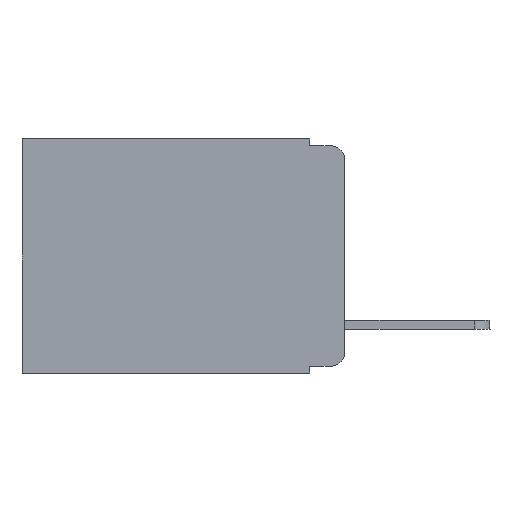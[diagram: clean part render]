
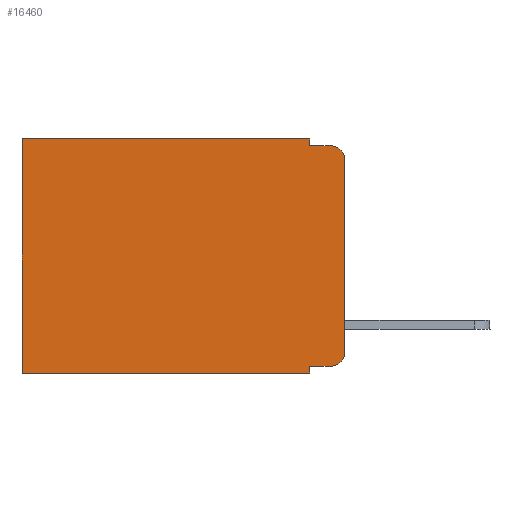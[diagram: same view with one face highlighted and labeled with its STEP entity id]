
A CAD part, left-side view. The second image highlights one B-rep face of the part: STEP entity #16460.
In plain terms, the highlighted planar face has unit normal (-1, 0, 0).
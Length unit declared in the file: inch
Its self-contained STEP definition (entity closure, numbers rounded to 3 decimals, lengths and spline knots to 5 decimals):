
#746 = CIRCLE ( 'NONE', #1974, 0.02 ) ;
#1625 = VERTEX_POINT ( 'NONE', #5108 ) ;
#1913 = CARTESIAN_POINT ( 'NONE',  ( 0.298, 0.02, -0.333 ) ) ;
#1974 = AXIS2_PLACEMENT_3D ( 'NONE', #5790, #13665, #3856 ) ;
#2011 = ORIENTED_EDGE ( 'NONE', *, *, #16342, .T. ) ;
#2152 = CARTESIAN_POINT ( 'NONE',  ( 0.298, 0.051, -0.01 ) ) ;
#2424 = ORIENTED_EDGE ( 'NONE', *, *, #23788, .T. ) ;
#2714 = VERTEX_POINT ( 'NONE', #8242 ) ;
#3777 = VECTOR ( 'NONE', #24983, 39.37008 ) ;
#3856 = DIRECTION ( 'NONE',  ( 0., 0., -1. ) ) ;
#3954 = VECTOR ( 'NONE', #24183, 39.37008 ) ;
#3997 = PLANE ( 'NONE',  #16964 ) ;
#4040 = CARTESIAN_POINT ( 'NONE',  ( 0.298, 0.473, 0. ) ) ;
#4423 = ORIENTED_EDGE ( 'NONE', *, *, #13741, .T. ) ;
#4662 = VECTOR ( 'NONE', #5682, 39.37008 ) ;
#5108 = CARTESIAN_POINT ( 'NONE',  ( 0.298, 0.473, -0.343 ) ) ;
#5442 = VERTEX_POINT ( 'NONE', #7423 ) ;
#5682 = DIRECTION ( 'NONE',  ( 0., -1., 0. ) ) ;
#5790 = CARTESIAN_POINT ( 'NONE',  ( 0.298, 0.02, -0.03 ) ) ;
#6003 = VERTEX_POINT ( 'NONE', #4040 ) ;
#6009 = VECTOR ( 'NONE', #10726, 39.37008 ) ;
#6402 = CIRCLE ( 'NONE', #9710, 0.02 ) ;
#6688 = CARTESIAN_POINT ( 'NONE',  ( 0.298, 0., 0. ) ) ;
#6774 = DIRECTION ( 'NONE',  ( 0., 0., -1. ) ) ;
#7169 = CARTESIAN_POINT ( 'NONE',  ( 0.298, 0., -0.03 ) ) ;
#7273 = VECTOR ( 'NONE', #11265, 39.37008 ) ;
#7423 = CARTESIAN_POINT ( 'NONE',  ( 0.298, 0.051, -0.343 ) ) ;
#7435 = CARTESIAN_POINT ( 'NONE',  ( 0.298, 0., -0.313 ) ) ;
#7509 = DIRECTION ( 'NONE',  ( 0., 0., -1. ) ) ;
#8242 = CARTESIAN_POINT ( 'NONE',  ( 0.298, 0.051, 0. ) ) ;
#8261 = LINE ( 'NONE', #24100, #6009 ) ;
#8814 = EDGE_CURVE ( 'NONE', #17631, #5442, #17061, .T. ) ;
#9164 = VECTOR ( 'NONE', #6774, 39.37008 ) ;
#9539 = FACE_OUTER_BOUND ( 'NONE', #16174, .T. ) ;
#9710 = AXIS2_PLACEMENT_3D ( 'NONE', #15259, #15136, #7509 ) ;
#9766 = CARTESIAN_POINT ( 'NONE',  ( 0.298, 0.02, -0.01 ) ) ;
#9841 = EDGE_CURVE ( 'NONE', #20473, #23531, #746, .T. ) ;
#10006 = LINE ( 'NONE', #14264, #21093 ) ;
#10542 = CARTESIAN_POINT ( 'NONE',  ( 0.298, 0., -0.343 ) ) ;
#10726 = DIRECTION ( 'NONE',  ( 0., 0., -1. ) ) ;
#11265 = DIRECTION ( 'NONE',  ( 0., 0., -1. ) ) ;
#11506 = VERTEX_POINT ( 'NONE', #2152 ) ;
#12406 = ORIENTED_EDGE ( 'NONE', *, *, #17165, .F. ) ;
#12609 = LINE ( 'NONE', #10542, #3954 ) ;
#12883 = LINE ( 'NONE', #6688, #21609 ) ;
#13665 = DIRECTION ( 'NONE',  ( -1., 0., 0. ) ) ;
#13741 = EDGE_CURVE ( 'NONE', #17631, #23526, #23322, .T. ) ;
#14264 = CARTESIAN_POINT ( 'NONE',  ( 0.298, 0.051, -0.01 ) ) ;
#14398 = EDGE_CURVE ( 'NONE', #11506, #23531, #10006, .T. ) ;
#14998 = CARTESIAN_POINT ( 'NONE',  ( 0.298, 0.051, -0.333 ) ) ;
#15136 = DIRECTION ( 'NONE',  ( -1., 0., 0. ) ) ;
#15259 = CARTESIAN_POINT ( 'NONE',  ( 0.298, 0.02, -0.313 ) ) ;
#16174 = EDGE_LOOP ( 'NONE', ( #12406, #21165, #24894, #22397, #22402, #2011, #18410, #25154, #4423, #2424 ) ) ;
#16342 = EDGE_CURVE ( 'NONE', #6003, #1625, #20889, .T. ) ;
#16460 = ADVANCED_FACE ( 'NONE', ( #9539 ), #3997, .F. ) ;
#16953 = LINE ( 'NONE', #22501, #9164 ) ;
#16964 = AXIS2_PLACEMENT_3D ( 'NONE', #19575, #19717, #17522 ) ;
#17061 = LINE ( 'NONE', #18997, #7273 ) ;
#17165 = EDGE_CURVE ( 'NONE', #20473, #21782, #16953, .T. ) ;
#17393 = CARTESIAN_POINT ( 'NONE',  ( 0.298, 0.051, -0.333 ) ) ;
#17522 = DIRECTION ( 'NONE',  ( 0., 0., -1. ) ) ;
#17631 = VERTEX_POINT ( 'NONE', #14998 ) ;
#18410 = ORIENTED_EDGE ( 'NONE', *, *, #20294, .F. ) ;
#18997 = CARTESIAN_POINT ( 'NONE',  ( 0.298, 0.051, 0. ) ) ;
#19575 = CARTESIAN_POINT ( 'NONE',  ( 0.298, 0., 0. ) ) ;
#19696 = EDGE_CURVE ( 'NONE', #2714, #6003, #12883, .T. ) ;
#19717 = DIRECTION ( 'NONE',  ( 1., 0., 0. ) ) ;
#20294 = EDGE_CURVE ( 'NONE', #5442, #1625, #12609, .T. ) ;
#20473 = VERTEX_POINT ( 'NONE', #7169 ) ;
#20889 = LINE ( 'NONE', #21012, #3777 ) ;
#21012 = CARTESIAN_POINT ( 'NONE',  ( 0.298, 0.473, 0. ) ) ;
#21093 = VECTOR ( 'NONE', #22116, 39.37008 ) ;
#21165 = ORIENTED_EDGE ( 'NONE', *, *, #9841, .T. ) ;
#21609 = VECTOR ( 'NONE', #22671, 39.37008 ) ;
#21782 = VERTEX_POINT ( 'NONE', #7435 ) ;
#22116 = DIRECTION ( 'NONE',  ( 0., -1., 0. ) ) ;
#22397 = ORIENTED_EDGE ( 'NONE', *, *, #24111, .F. ) ;
#22402 = ORIENTED_EDGE ( 'NONE', *, *, #19696, .T. ) ;
#22501 = CARTESIAN_POINT ( 'NONE',  ( 0.298, 0., 0. ) ) ;
#22671 = DIRECTION ( 'NONE',  ( 0., 1., 0. ) ) ;
#23322 = LINE ( 'NONE', #17393, #4662 ) ;
#23526 = VERTEX_POINT ( 'NONE', #1913 ) ;
#23531 = VERTEX_POINT ( 'NONE', #9766 ) ;
#23788 = EDGE_CURVE ( 'NONE', #23526, #21782, #6402, .T. ) ;
#24100 = CARTESIAN_POINT ( 'NONE',  ( 0.298, 0.051, 0. ) ) ;
#24111 = EDGE_CURVE ( 'NONE', #2714, #11506, #8261, .T. ) ;
#24183 = DIRECTION ( 'NONE',  ( 0., 1., 0. ) ) ;
#24894 = ORIENTED_EDGE ( 'NONE', *, *, #14398, .F. ) ;
#24983 = DIRECTION ( 'NONE',  ( 0., 0., -1. ) ) ;
#25154 = ORIENTED_EDGE ( 'NONE', *, *, #8814, .F. ) ;
